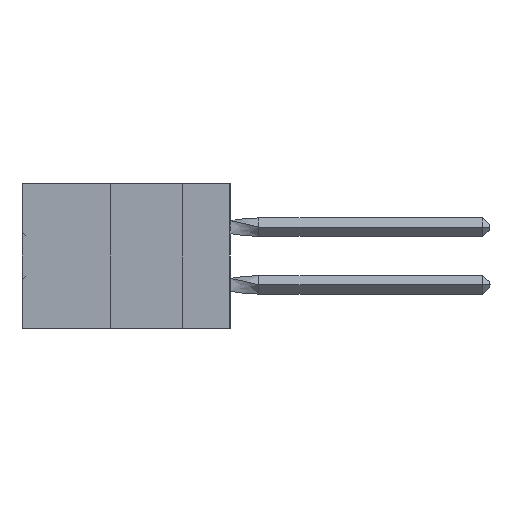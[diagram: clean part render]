
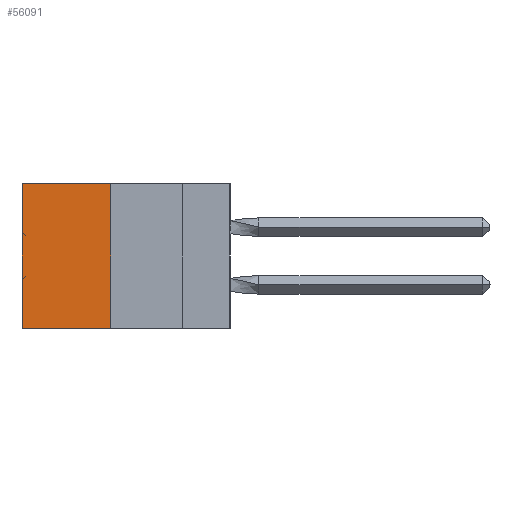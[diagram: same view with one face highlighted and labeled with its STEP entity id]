
A CAD part, left-side view. The second image highlights one B-rep face of the part: STEP entity #56091.
In plain terms, the highlighted planar face has unit normal (-1, 0, 0).
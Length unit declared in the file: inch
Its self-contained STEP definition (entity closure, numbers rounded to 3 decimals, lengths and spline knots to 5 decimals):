
#829 = VECTOR ( 'NONE', #19896, 39.37008 ) ;
#1231 = EDGE_CURVE ( 'NONE', #56169, #45761, #1585, .T. ) ;
#1585 = LINE ( 'NONE', #34081, #829 ) ;
#2946 = DIRECTION ( 'NONE',  ( 0., 1., 0. ) ) ;
#4268 = CARTESIAN_POINT ( 'NONE',  ( 0.305, 0.72, -0.5 ) ) ;
#12549 = LINE ( 'NONE', #44954, #38901 ) ;
#19896 = DIRECTION ( 'NONE',  ( 0., 0., -1. ) ) ;
#22569 = DIRECTION ( 'NONE',  ( 1., 0., 0. ) ) ;
#23752 = CARTESIAN_POINT ( 'NONE',  ( 0.305, 0.413, -0.5 ) ) ;
#23876 = VERTEX_POINT ( 'NONE', #52220 ) ;
#30014 = ORIENTED_EDGE ( 'NONE', *, *, #1231, .F. ) ;
#30705 = CARTESIAN_POINT ( 'NONE',  ( 0.305, 0.413, 0. ) ) ;
#33454 = CARTESIAN_POINT ( 'NONE',  ( 0.305, 0.72, -0.5 ) ) ;
#33678 = DIRECTION ( 'NONE',  ( 0., 0., -1. ) ) ;
#34081 = CARTESIAN_POINT ( 'NONE',  ( 0.305, 0.413, -0.5 ) ) ;
#35416 = ORIENTED_EDGE ( 'NONE', *, *, #49219, .T. ) ;
#36426 = EDGE_LOOP ( 'NONE', ( #43998, #57663, #30014, #35416 ) ) ;
#36469 = VECTOR ( 'NONE', #33678, 39.37008 ) ;
#36720 = PLANE ( 'NONE',  #54032 ) ;
#38901 = VECTOR ( 'NONE', #2946, 39.37008 ) ;
#39716 = DIRECTION ( 'NONE',  ( 0., 1., 0. ) ) ;
#42476 = VERTEX_POINT ( 'NONE', #4268 ) ;
#43998 = ORIENTED_EDGE ( 'NONE', *, *, #55009, .T. ) ;
#44954 = CARTESIAN_POINT ( 'NONE',  ( 0.305, 0.413, -0.5 ) ) ;
#45761 = VERTEX_POINT ( 'NONE', #23752 ) ;
#46190 = DIRECTION ( 'NONE',  ( 0., 0., -1. ) ) ;
#49219 = EDGE_CURVE ( 'NONE', #56169, #23876, #52560, .T. ) ;
#50655 = CARTESIAN_POINT ( 'NONE',  ( 0.305, 0.413, -0.5 ) ) ;
#52057 = CARTESIAN_POINT ( 'NONE',  ( 0.305, 0.413, 0. ) ) ;
#52220 = CARTESIAN_POINT ( 'NONE',  ( 0.305, 0.72, 0. ) ) ;
#52560 = LINE ( 'NONE', #30705, #59895 ) ;
#53166 = FACE_OUTER_BOUND ( 'NONE', #36426, .T. ) ;
#54032 = AXIS2_PLACEMENT_3D ( 'NONE', #50655, #22569, #46190 ) ;
#54816 = LINE ( 'NONE', #33454, #36469 ) ;
#55009 = EDGE_CURVE ( 'NONE', #23876, #42476, #54816, .T. ) ;
#56091 = ADVANCED_FACE ( 'NONE', ( #53166 ), #36720, .F. ) ;
#56169 = VERTEX_POINT ( 'NONE', #52057 ) ;
#57663 = ORIENTED_EDGE ( 'NONE', *, *, #59245, .F. ) ;
#59245 = EDGE_CURVE ( 'NONE', #45761, #42476, #12549, .T. ) ;
#59895 = VECTOR ( 'NONE', #39716, 39.37008 ) ;
